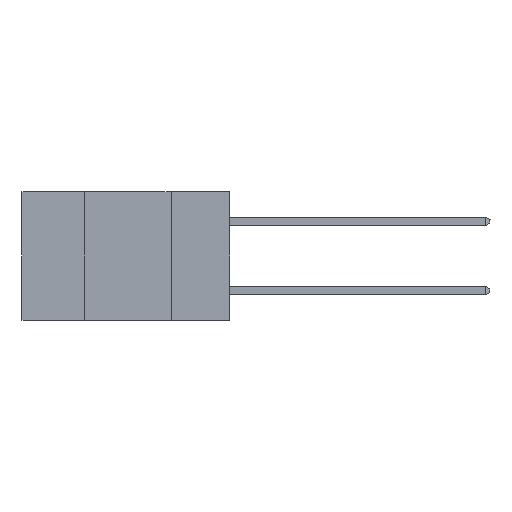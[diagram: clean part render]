
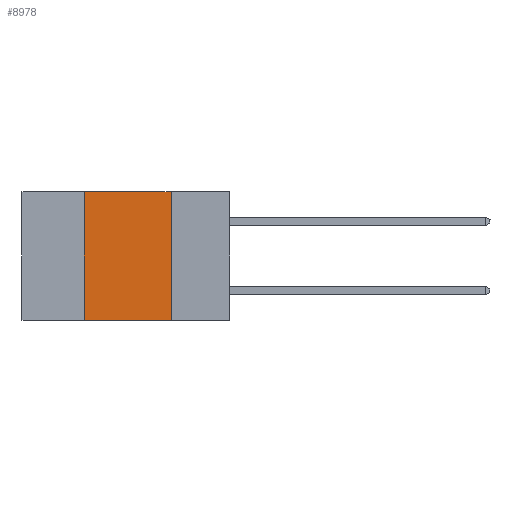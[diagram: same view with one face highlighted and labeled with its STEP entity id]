
A CAD part, left-side view. The second image highlights one B-rep face of the part: STEP entity #8978.
In plain terms, the highlighted planar face has unit normal (-1, 0, 0).
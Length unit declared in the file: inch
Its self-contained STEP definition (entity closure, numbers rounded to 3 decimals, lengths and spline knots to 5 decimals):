
#229 = VERTEX_POINT ( 'NONE', #5660 ) ;
#272 = EDGE_LOOP ( 'NONE', ( #4944, #8089, #9128, #7269 ) ) ;
#619 = VERTEX_POINT ( 'NONE', #2114 ) ;
#1011 = VECTOR ( 'NONE', #2523, 39.37008 ) ;
#2056 = DIRECTION ( 'NONE',  ( 0., 0., -1. ) ) ;
#2114 = CARTESIAN_POINT ( 'NONE',  ( 0., 0.42, -0.37 ) ) ;
#2170 = DIRECTION ( 'NONE',  ( 0., 0., 1. ) ) ;
#2523 = DIRECTION ( 'NONE',  ( 0., -1., 0. ) ) ;
#2634 = VECTOR ( 'NONE', #6305, 39.37008 ) ;
#3036 = EDGE_CURVE ( 'NONE', #10349, #229, #3853, .T. ) ;
#3123 = CARTESIAN_POINT ( 'NONE',  ( 0., 0.6, 0. ) ) ;
#3298 = VERTEX_POINT ( 'NONE', #8081 ) ;
#3540 = EDGE_CURVE ( 'NONE', #229, #3298, #7796, .T. ) ;
#3763 = AXIS2_PLACEMENT_3D ( 'NONE', #3123, #9614, #8846 ) ;
#3853 = LINE ( 'NONE', #8804, #2634 ) ;
#4461 = VECTOR ( 'NONE', #2056, 39.37008 ) ;
#4932 = EDGE_CURVE ( 'NONE', #619, #10349, #9634, .T. ) ;
#4944 = ORIENTED_EDGE ( 'NONE', *, *, #3540, .F. ) ;
#5408 = EDGE_CURVE ( 'NONE', #619, #3298, #8132, .T. ) ;
#5592 = PLANE ( 'NONE',  #3763 ) ;
#5660 = CARTESIAN_POINT ( 'NONE',  ( 0., 0.17, 0. ) ) ;
#6305 = DIRECTION ( 'NONE',  ( 0., -1., 0. ) ) ;
#6893 = VECTOR ( 'NONE', #2170, 39.37008 ) ;
#7269 = ORIENTED_EDGE ( 'NONE', *, *, #5408, .T. ) ;
#7796 = LINE ( 'NONE', #9669, #4461 ) ;
#8081 = CARTESIAN_POINT ( 'NONE',  ( 0., 0.17, -0.37 ) ) ;
#8089 = ORIENTED_EDGE ( 'NONE', *, *, #3036, .F. ) ;
#8132 = LINE ( 'NONE', #9219, #1011 ) ;
#8804 = CARTESIAN_POINT ( 'NONE',  ( 0., 0.6, 0. ) ) ;
#8846 = DIRECTION ( 'NONE',  ( 0., 0., -1. ) ) ;
#8978 = ADVANCED_FACE ( 'NONE', ( #10434 ), #5592, .F. ) ;
#9128 = ORIENTED_EDGE ( 'NONE', *, *, #4932, .F. ) ;
#9219 = CARTESIAN_POINT ( 'NONE',  ( 0., 0.6, -0.37 ) ) ;
#9576 = CARTESIAN_POINT ( 'NONE',  ( 0., 0.42, 0. ) ) ;
#9614 = DIRECTION ( 'NONE',  ( 1., 0., 0. ) ) ;
#9634 = LINE ( 'NONE', #10455, #6893 ) ;
#9669 = CARTESIAN_POINT ( 'NONE',  ( 0., 0.17, -0.37 ) ) ;
#10349 = VERTEX_POINT ( 'NONE', #9576 ) ;
#10434 = FACE_OUTER_BOUND ( 'NONE', #272, .T. ) ;
#10455 = CARTESIAN_POINT ( 'NONE',  ( 0., 0.42, -0.37 ) ) ;
